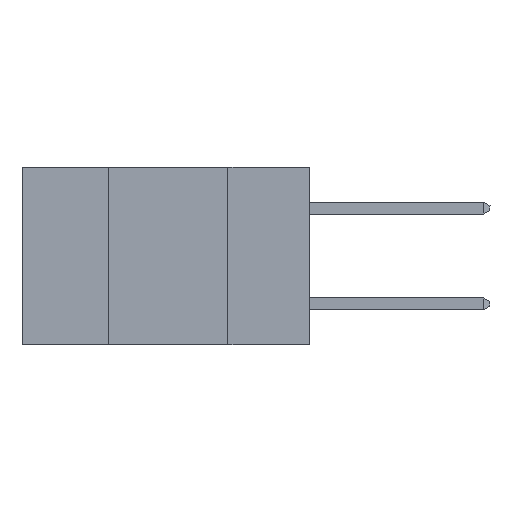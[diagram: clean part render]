
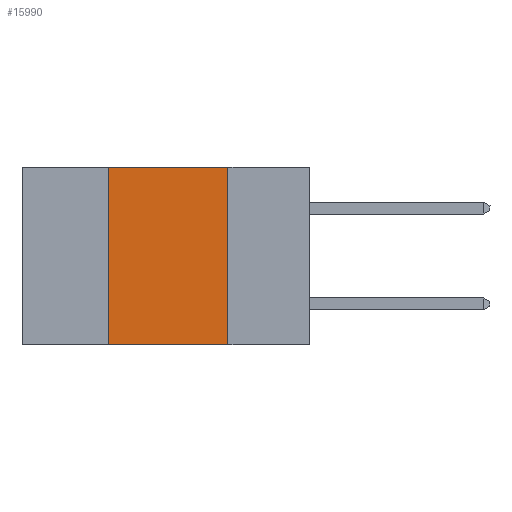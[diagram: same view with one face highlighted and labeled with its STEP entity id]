
A CAD part, left-side view. The second image highlights one B-rep face of the part: STEP entity #15990.
In plain terms, the highlighted planar face has unit normal (-1, 0, 0).
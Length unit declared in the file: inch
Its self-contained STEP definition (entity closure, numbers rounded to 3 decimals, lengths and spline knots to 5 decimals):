
#575 = EDGE_CURVE ( 'NONE', #11033, #12312, #16519, .T. ) ;
#1555 = DIRECTION ( 'NONE',  ( 0., 0., -1. ) ) ;
#1741 = ORIENTED_EDGE ( 'NONE', *, *, #15261, .F. ) ;
#1805 = LINE ( 'NONE', #8869, #5232 ) ;
#2801 = LINE ( 'NONE', #5374, #12643 ) ;
#2860 = VECTOR ( 'NONE', #12044, 39.37008 ) ;
#3449 = AXIS2_PLACEMENT_3D ( 'NONE', #4892, #13898, #6182 ) ;
#4885 = CARTESIAN_POINT ( 'NONE',  ( 0., 0.42, 0. ) ) ;
#4892 = CARTESIAN_POINT ( 'NONE',  ( 0., 0.6, 0. ) ) ;
#5032 = DIRECTION ( 'NONE',  ( 0., -1., 0. ) ) ;
#5232 = VECTOR ( 'NONE', #5032, 39.37008 ) ;
#5374 = CARTESIAN_POINT ( 'NONE',  ( 0., 0.17, 0. ) ) ;
#6041 = VERTEX_POINT ( 'NONE', #9923 ) ;
#6178 = VECTOR ( 'NONE', #15523, 39.37008 ) ;
#6182 = DIRECTION ( 'NONE',  ( 0., 0., -1. ) ) ;
#7611 = CARTESIAN_POINT ( 'NONE',  ( 0., 0.17, -0.37 ) ) ;
#8126 = VERTEX_POINT ( 'NONE', #7611 ) ;
#8340 = EDGE_LOOP ( 'NONE', ( #13094, #1741, #10018, #12390 ) ) ;
#8726 = PLANE ( 'NONE',  #3449 ) ;
#8869 = CARTESIAN_POINT ( 'NONE',  ( 0., 0.6, 0. ) ) ;
#9040 = CARTESIAN_POINT ( 'NONE',  ( 0., 0.42, 0. ) ) ;
#9923 = CARTESIAN_POINT ( 'NONE',  ( 0., 0.17, 0. ) ) ;
#10018 = ORIENTED_EDGE ( 'NONE', *, *, #575, .F. ) ;
#10024 = LINE ( 'NONE', #14244, #6178 ) ;
#10246 = FACE_OUTER_BOUND ( 'NONE', #8340, .T. ) ;
#11033 = VERTEX_POINT ( 'NONE', #11307 ) ;
#11307 = CARTESIAN_POINT ( 'NONE',  ( 0., 0.42, -0.37 ) ) ;
#12044 = DIRECTION ( 'NONE',  ( 0., 0., 1. ) ) ;
#12312 = VERTEX_POINT ( 'NONE', #4885 ) ;
#12390 = ORIENTED_EDGE ( 'NONE', *, *, #12882, .T. ) ;
#12643 = VECTOR ( 'NONE', #1555, 39.37008 ) ;
#12882 = EDGE_CURVE ( 'NONE', #11033, #8126, #10024, .T. ) ;
#13094 = ORIENTED_EDGE ( 'NONE', *, *, #16275, .F. ) ;
#13898 = DIRECTION ( 'NONE',  ( 1., 0., 0. ) ) ;
#14244 = CARTESIAN_POINT ( 'NONE',  ( 0., 0.6, -0.37 ) ) ;
#15261 = EDGE_CURVE ( 'NONE', #12312, #6041, #1805, .T. ) ;
#15523 = DIRECTION ( 'NONE',  ( 0., -1., 0. ) ) ;
#15990 = ADVANCED_FACE ( 'NONE', ( #10246 ), #8726, .F. ) ;
#16275 = EDGE_CURVE ( 'NONE', #6041, #8126, #2801, .T. ) ;
#16519 = LINE ( 'NONE', #9040, #2860 ) ;
